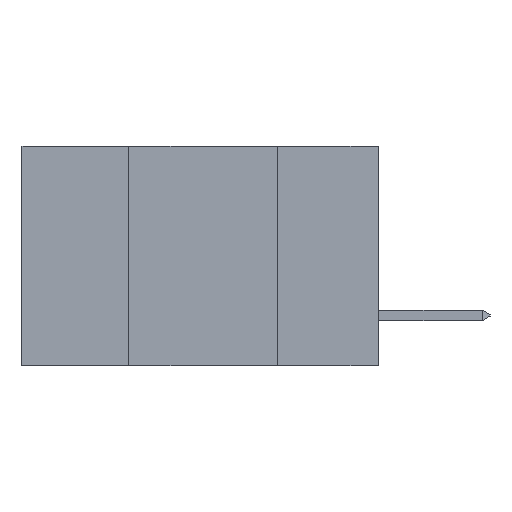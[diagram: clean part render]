
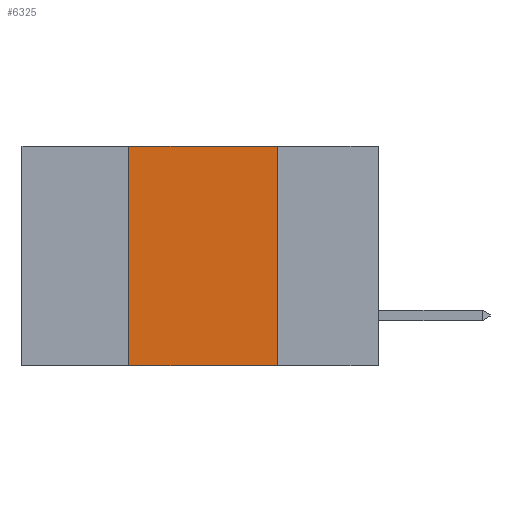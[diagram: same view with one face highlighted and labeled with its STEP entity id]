
A CAD part, left-side view. The second image highlights one B-rep face of the part: STEP entity #6325.
In plain terms, the highlighted planar face has unit normal (-1, 0, 0).
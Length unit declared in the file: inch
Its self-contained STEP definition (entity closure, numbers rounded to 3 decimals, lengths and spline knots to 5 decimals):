
#237 = CARTESIAN_POINT ( 'NONE',  ( 0., 0.6, 0. ) ) ;
#2252 = CARTESIAN_POINT ( 'NONE',  ( 0., 0.42, 0. ) ) ;
#2768 = FACE_OUTER_BOUND ( 'NONE', #14635, .T. ) ;
#3527 = ORIENTED_EDGE ( 'NONE', *, *, #5665, .T. ) ;
#4749 = CARTESIAN_POINT ( 'NONE',  ( 0., 0.42, 0. ) ) ;
#4770 = LINE ( 'NONE', #8554, #16602 ) ;
#5665 = EDGE_CURVE ( 'NONE', #12969, #14356, #17449, .T. ) ;
#6299 = LINE ( 'NONE', #4749, #9843 ) ;
#6325 = ADVANCED_FACE ( 'NONE', ( #2768 ), #11030, .F. ) ;
#6572 = VERTEX_POINT ( 'NONE', #16640 ) ;
#7705 = VERTEX_POINT ( 'NONE', #2252 ) ;
#8430 = ORIENTED_EDGE ( 'NONE', *, *, #11286, .F. ) ;
#8554 = CARTESIAN_POINT ( 'NONE',  ( 0., 0.17, 0. ) ) ;
#9843 = VECTOR ( 'NONE', #15149, 39.37008 ) ;
#9882 = DIRECTION ( 'NONE',  ( 0., -1., 0. ) ) ;
#10158 = CARTESIAN_POINT ( 'NONE',  ( 0., 0.17, -0.37 ) ) ;
#10411 = ORIENTED_EDGE ( 'NONE', *, *, #15655, .F. ) ;
#10418 = LINE ( 'NONE', #237, #17785 ) ;
#11030 = PLANE ( 'NONE',  #15604 ) ;
#11160 = DIRECTION ( 'NONE',  ( 1., 0., 0. ) ) ;
#11286 = EDGE_CURVE ( 'NONE', #7705, #6572, #10418, .T. ) ;
#11435 = DIRECTION ( 'NONE',  ( 0., 0., -1. ) ) ;
#12969 = VERTEX_POINT ( 'NONE', #14082 ) ;
#14001 = VECTOR ( 'NONE', #9882, 39.37008 ) ;
#14082 = CARTESIAN_POINT ( 'NONE',  ( 0., 0.42, -0.37 ) ) ;
#14356 = VERTEX_POINT ( 'NONE', #10158 ) ;
#14635 = EDGE_LOOP ( 'NONE', ( #17558, #8430, #10411, #3527 ) ) ;
#14693 = EDGE_CURVE ( 'NONE', #6572, #14356, #4770, .T. ) ;
#15011 = DIRECTION ( 'NONE',  ( 0., -1., 0. ) ) ;
#15149 = DIRECTION ( 'NONE',  ( 0., 0., 1. ) ) ;
#15203 = CARTESIAN_POINT ( 'NONE',  ( 0., 0.6, -0.37 ) ) ;
#15604 = AXIS2_PLACEMENT_3D ( 'NONE', #16662, #11160, #11435 ) ;
#15655 = EDGE_CURVE ( 'NONE', #12969, #7705, #6299, .T. ) ;
#16602 = VECTOR ( 'NONE', #17418, 39.37008 ) ;
#16640 = CARTESIAN_POINT ( 'NONE',  ( 0., 0.17, 0. ) ) ;
#16662 = CARTESIAN_POINT ( 'NONE',  ( 0., 0.6, 0. ) ) ;
#17418 = DIRECTION ( 'NONE',  ( 0., 0., -1. ) ) ;
#17449 = LINE ( 'NONE', #15203, #14001 ) ;
#17558 = ORIENTED_EDGE ( 'NONE', *, *, #14693, .F. ) ;
#17785 = VECTOR ( 'NONE', #15011, 39.37008 ) ;
